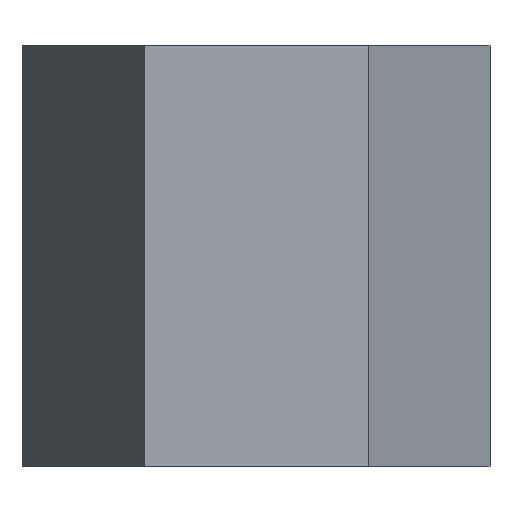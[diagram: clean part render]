
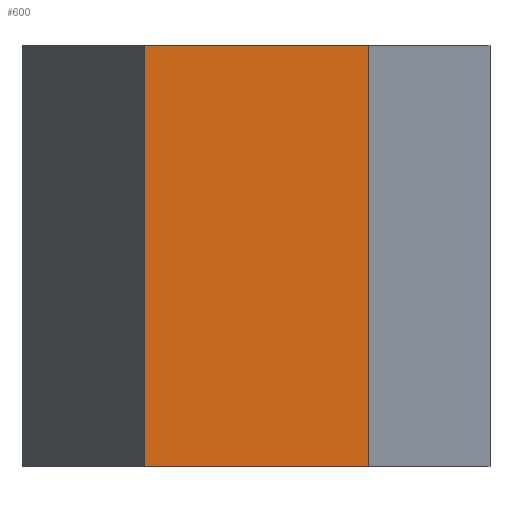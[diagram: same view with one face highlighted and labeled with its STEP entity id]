
A CAD part, left-side view. The second image highlights one B-rep face of the part: STEP entity #600.
In plain terms, the highlighted planar face has unit normal (-1, 0, 0).
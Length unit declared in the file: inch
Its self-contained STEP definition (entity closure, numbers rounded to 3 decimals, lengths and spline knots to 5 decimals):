
#9 = DIRECTION ( 'NONE',  ( 0., 0., 1. ) ) ;
#39 = ORIENTED_EDGE ( 'NONE', *, *, #217, .T. ) ;
#68 = ORIENTED_EDGE ( 'NONE', *, *, #169, .T. ) ;
#71 = CARTESIAN_POINT ( 'NONE',  ( -0.75, 0.38, 0.14 ) ) ;
#95 = LINE ( 'NONE', #649, #112 ) ;
#107 = FACE_OUTER_BOUND ( 'NONE', #409, .T. ) ;
#112 = VECTOR ( 'NONE', #9, 39.37008 ) ;
#122 = CARTESIAN_POINT ( 'NONE',  ( -0.75, 1.08, 1.455 ) ) ;
#161 = VERTEX_POINT ( 'NONE', #122 ) ;
#169 = EDGE_CURVE ( 'NONE', #238, #252, #442, .T. ) ;
#179 = ORIENTED_EDGE ( 'NONE', *, *, #598, .F. ) ;
#187 = LINE ( 'NONE', #198, #196 ) ;
#196 = VECTOR ( 'NONE', #525, 39.37008 ) ;
#198 = CARTESIAN_POINT ( 'NONE',  ( -0.75, 0.38, 0.14 ) ) ;
#217 = EDGE_CURVE ( 'NONE', #252, #161, #463, .T. ) ;
#233 = CARTESIAN_POINT ( 'NONE',  ( -0.75, 0.38, 0.14 ) ) ;
#238 = VERTEX_POINT ( 'NONE', #233 ) ;
#252 = VERTEX_POINT ( 'NONE', #618 ) ;
#363 = VECTOR ( 'NONE', #440, 39.37008 ) ;
#381 = DIRECTION ( 'NONE',  ( 0., 0., 1. ) ) ;
#409 = EDGE_LOOP ( 'NONE', ( #68, #39, #179, #597 ) ) ;
#426 = CARTESIAN_POINT ( 'NONE',  ( -0.75, 1.08, 0.14 ) ) ;
#440 = DIRECTION ( 'NONE',  ( 0., 1., 0. ) ) ;
#442 = LINE ( 'NONE', #71, #465 ) ;
#448 = EDGE_CURVE ( 'NONE', #238, #655, #187, .T. ) ;
#463 = LINE ( 'NONE', #612, #363 ) ;
#465 = VECTOR ( 'NONE', #381, 39.37008 ) ;
#525 = DIRECTION ( 'NONE',  ( 0., 1., 0. ) ) ;
#583 = DIRECTION ( 'NONE',  ( 0., 1., 0. ) ) ;
#590 = DIRECTION ( 'NONE',  ( -1., 0., 0. ) ) ;
#593 = PLANE ( 'NONE',  #642 ) ;
#597 = ORIENTED_EDGE ( 'NONE', *, *, #448, .F. ) ;
#598 = EDGE_CURVE ( 'NONE', #655, #161, #95, .T. ) ;
#600 = ADVANCED_FACE ( 'NONE', ( #107 ), #593, .T. ) ;
#604 = CARTESIAN_POINT ( 'NONE',  ( -0.75, 0.38, 0. ) ) ;
#612 = CARTESIAN_POINT ( 'NONE',  ( -0.75, 0.38, 1.455 ) ) ;
#618 = CARTESIAN_POINT ( 'NONE',  ( -0.75, 0.38, 1.455 ) ) ;
#642 = AXIS2_PLACEMENT_3D ( 'NONE', #604, #590, #583 ) ;
#649 = CARTESIAN_POINT ( 'NONE',  ( -0.75, 1.08, 0.14 ) ) ;
#655 = VERTEX_POINT ( 'NONE', #426 ) ;
